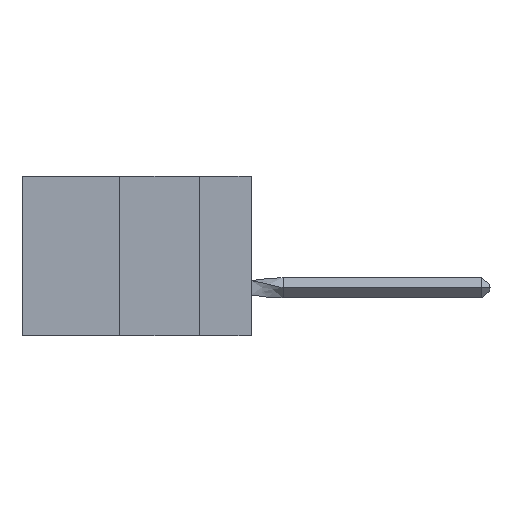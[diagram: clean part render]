
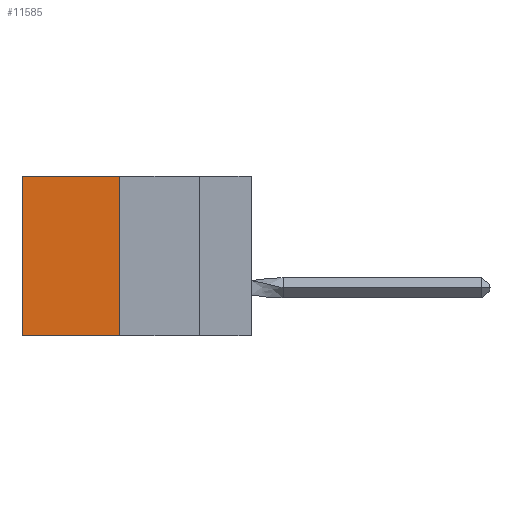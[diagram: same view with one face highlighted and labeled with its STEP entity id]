
A CAD part, left-side view. The second image highlights one B-rep face of the part: STEP entity #11585.
In plain terms, the highlighted planar face has unit normal (-1, 0, 0).
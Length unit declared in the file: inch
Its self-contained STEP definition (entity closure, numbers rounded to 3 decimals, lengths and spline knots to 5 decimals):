
#755 = VERTEX_POINT ( 'NONE', #5126 ) ;
#1853 = EDGE_LOOP ( 'NONE', ( #3624, #21001, #3619, #19116 ) ) ;
#1989 = CARTESIAN_POINT ( 'NONE',  ( 0.305, 0.413, -0.5 ) ) ;
#2671 = VECTOR ( 'NONE', #7649, 39.37008 ) ;
#3619 = ORIENTED_EDGE ( 'NONE', *, *, #5119, .F. ) ;
#3624 = ORIENTED_EDGE ( 'NONE', *, *, #12405, .T. ) ;
#4401 = CARTESIAN_POINT ( 'NONE',  ( 0.305, 0.72, 0. ) ) ;
#4723 = LINE ( 'NONE', #1989, #15022 ) ;
#5046 = CARTESIAN_POINT ( 'NONE',  ( 0.305, 0.413, -0.5 ) ) ;
#5112 = PLANE ( 'NONE',  #19176 ) ;
#5119 = EDGE_CURVE ( 'NONE', #8944, #14698, #4723, .T. ) ;
#5126 = CARTESIAN_POINT ( 'NONE',  ( 0.305, 0.72, -0.5 ) ) ;
#5882 = EDGE_CURVE ( 'NONE', #8944, #20673, #12141, .T. ) ;
#6344 = FACE_OUTER_BOUND ( 'NONE', #1853, .T. ) ;
#6904 = EDGE_CURVE ( 'NONE', #14698, #755, #16550, .T. ) ;
#7649 = DIRECTION ( 'NONE',  ( 0., 0., -1. ) ) ;
#8514 = DIRECTION ( 'NONE',  ( 0., 1., 0. ) ) ;
#8944 = VERTEX_POINT ( 'NONE', #18774 ) ;
#9335 = CARTESIAN_POINT ( 'NONE',  ( 0.305, 0.413, 0. ) ) ;
#10189 = DIRECTION ( 'NONE',  ( 1., 0., 0. ) ) ;
#10756 = DIRECTION ( 'NONE',  ( 0., 1., 0. ) ) ;
#11585 = ADVANCED_FACE ( 'NONE', ( #6344 ), #5112, .F. ) ;
#12141 = LINE ( 'NONE', #9335, #16783 ) ;
#12405 = EDGE_CURVE ( 'NONE', #20673, #755, #15829, .T. ) ;
#14281 = CARTESIAN_POINT ( 'NONE',  ( 0.305, 0.72, -0.5 ) ) ;
#14698 = VERTEX_POINT ( 'NONE', #19753 ) ;
#14917 = CARTESIAN_POINT ( 'NONE',  ( 0.305, 0.413, -0.5 ) ) ;
#15022 = VECTOR ( 'NONE', #19769, 39.37008 ) ;
#15829 = LINE ( 'NONE', #14281, #2671 ) ;
#16550 = LINE ( 'NONE', #14917, #17821 ) ;
#16614 = DIRECTION ( 'NONE',  ( 0., 0., -1. ) ) ;
#16783 = VECTOR ( 'NONE', #10756, 39.37008 ) ;
#17821 = VECTOR ( 'NONE', #8514, 39.37008 ) ;
#18774 = CARTESIAN_POINT ( 'NONE',  ( 0.305, 0.413, 0. ) ) ;
#19116 = ORIENTED_EDGE ( 'NONE', *, *, #5882, .T. ) ;
#19176 = AXIS2_PLACEMENT_3D ( 'NONE', #5046, #10189, #16614 ) ;
#19753 = CARTESIAN_POINT ( 'NONE',  ( 0.305, 0.413, -0.5 ) ) ;
#19769 = DIRECTION ( 'NONE',  ( 0., 0., -1. ) ) ;
#20673 = VERTEX_POINT ( 'NONE', #4401 ) ;
#21001 = ORIENTED_EDGE ( 'NONE', *, *, #6904, .F. ) ;
